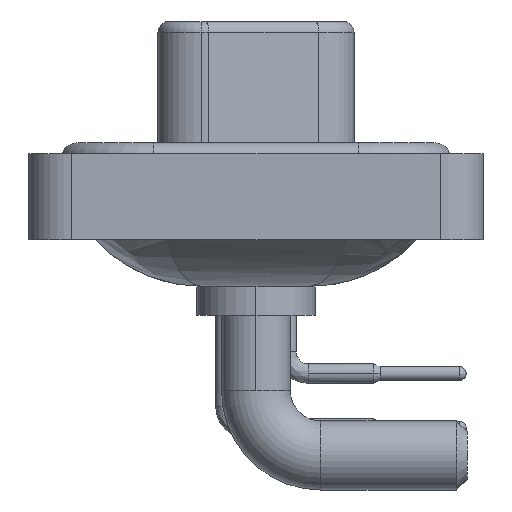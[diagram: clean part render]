
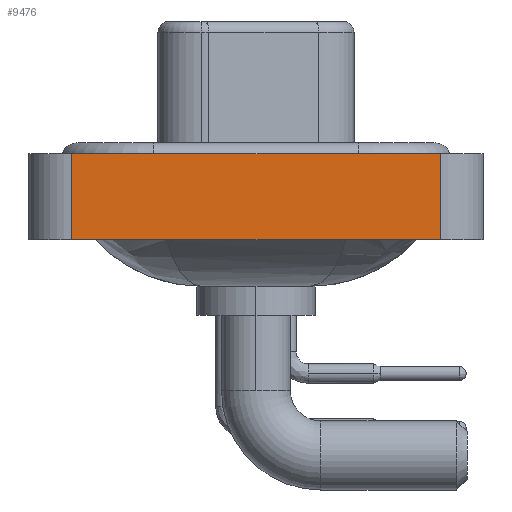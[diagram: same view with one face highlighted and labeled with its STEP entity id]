
A CAD part, left-side view. The second image highlights one B-rep face of the part: STEP entity #9476.
In plain terms, the highlighted planar face has unit normal (-1, 0, 0).
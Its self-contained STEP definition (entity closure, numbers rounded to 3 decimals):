
#752 = CARTESIAN_POINT ( 'NONE',  ( -7.35, -8.55, -3.6 ) ) ;
#1084 = DIRECTION ( 'NONE',  ( 0., 0., 1. ) ) ;
#1231 = ORIENTED_EDGE ( 'NONE', *, *, #10043, .F. ) ;
#1931 = LINE ( 'NONE', #10699, #15169 ) ;
#2134 = VECTOR ( 'NONE', #6565, 1000. ) ;
#2796 = CARTESIAN_POINT ( 'NONE',  ( -7.35, -8.55, -3.6 ) ) ;
#5076 = EDGE_CURVE ( 'NONE', #24709, #14495, #13707, .T. ) ;
#5982 = DIRECTION ( 'NONE',  ( -1., 0., 0. ) ) ;
#6565 = DIRECTION ( 'NONE',  ( 0., 0., 1. ) ) ;
#6579 = VERTEX_POINT ( 'NONE', #8435 ) ;
#6867 = ORIENTED_EDGE ( 'NONE', *, *, #5076, .T. ) ;
#7897 = ORIENTED_EDGE ( 'NONE', *, *, #13462, .F. ) ;
#8062 = VECTOR ( 'NONE', #11824, 1000. ) ;
#8435 = CARTESIAN_POINT ( 'NONE',  ( -7.35, 8.55, 0.4 ) ) ;
#9476 = ADVANCED_FACE ( 'NONE', ( #27518 ), #10293, .T. ) ;
#10043 = EDGE_CURVE ( 'NONE', #6579, #21949, #1931, .T. ) ;
#10293 = PLANE ( 'NONE',  #22981 ) ;
#10699 = CARTESIAN_POINT ( 'NONE',  ( -7.35, -8.55, 0.4 ) ) ;
#10710 = EDGE_LOOP ( 'NONE', ( #15401, #1231, #7897, #6867 ) ) ;
#11824 = DIRECTION ( 'NONE',  ( 0., -1., 0. ) ) ;
#12871 = LINE ( 'NONE', #23897, #19089 ) ;
#13462 = EDGE_CURVE ( 'NONE', #24709, #6579, #17501, .T. ) ;
#13707 = LINE ( 'NONE', #2796, #8062 ) ;
#14495 = VERTEX_POINT ( 'NONE', #752 ) ;
#14859 = EDGE_CURVE ( 'NONE', #14495, #21949, #12871, .T. ) ;
#15169 = VECTOR ( 'NONE', #19172, 1000. ) ;
#15271 = CARTESIAN_POINT ( 'NONE',  ( -7.35, 8.55, -3.6 ) ) ;
#15401 = ORIENTED_EDGE ( 'NONE', *, *, #14859, .T. ) ;
#15725 = DIRECTION ( 'NONE',  ( 0., 0., 1. ) ) ;
#17501 = LINE ( 'NONE', #17636, #2134 ) ;
#17636 = CARTESIAN_POINT ( 'NONE',  ( -7.35, 8.55, -3.6 ) ) ;
#19089 = VECTOR ( 'NONE', #15725, 1000. ) ;
#19172 = DIRECTION ( 'NONE',  ( 0., -1., 0. ) ) ;
#21949 = VERTEX_POINT ( 'NONE', #24215 ) ;
#22981 = AXIS2_PLACEMENT_3D ( 'NONE', #23349, #5982, #1084 ) ;
#23349 = CARTESIAN_POINT ( 'NONE',  ( -7.35, -8.55, -3.6 ) ) ;
#23897 = CARTESIAN_POINT ( 'NONE',  ( -7.35, -8.55, -3.6 ) ) ;
#24215 = CARTESIAN_POINT ( 'NONE',  ( -7.35, -8.55, 0.4 ) ) ;
#24709 = VERTEX_POINT ( 'NONE', #15271 ) ;
#27518 = FACE_OUTER_BOUND ( 'NONE', #10710, .T. ) ;
